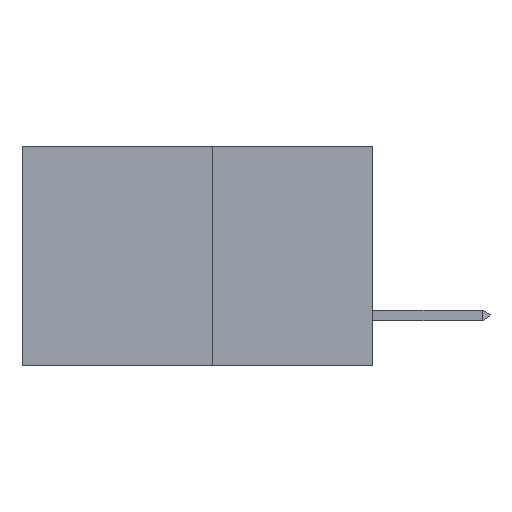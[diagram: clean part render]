
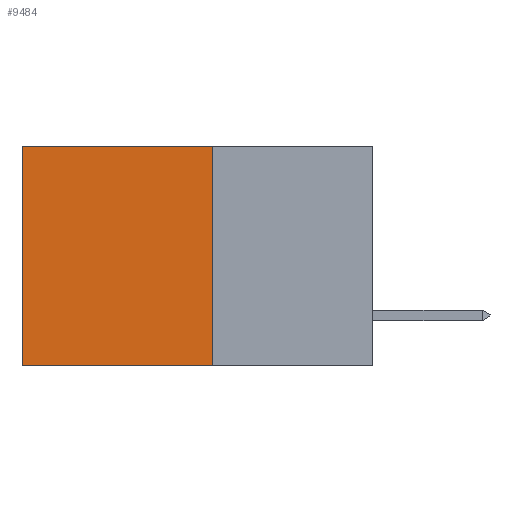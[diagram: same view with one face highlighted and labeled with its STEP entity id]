
A CAD part, left-side view. The second image highlights one B-rep face of the part: STEP entity #9484.
In plain terms, the highlighted planar face has unit normal (-1, 0, 0).
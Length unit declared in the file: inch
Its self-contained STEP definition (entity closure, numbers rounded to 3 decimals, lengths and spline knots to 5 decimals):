
#1274 = VERTEX_POINT ( 'NONE', #1843 ) ;
#1649 = DIRECTION ( 'NONE',  ( 0., 0., -1. ) ) ;
#1843 = CARTESIAN_POINT ( 'NONE',  ( 0.277, 0.59, 0. ) ) ;
#2267 = ORIENTED_EDGE ( 'NONE', *, *, #2368, .T. ) ;
#2368 = EDGE_CURVE ( 'NONE', #1274, #11305, #2535, .T. ) ;
#2535 = LINE ( 'NONE', #3333, #8054 ) ;
#2747 = CARTESIAN_POINT ( 'NONE',  ( 0.277, 0.27, -0.37 ) ) ;
#3224 = VECTOR ( 'NONE', #6146, 39.37008 ) ;
#3256 = DIRECTION ( 'NONE',  ( 0., 0., -1. ) ) ;
#3333 = CARTESIAN_POINT ( 'NONE',  ( 0.277, 0.59, -0.37 ) ) ;
#3532 = ORIENTED_EDGE ( 'NONE', *, *, #5782, .F. ) ;
#3908 = PLANE ( 'NONE',  #11185 ) ;
#4056 = CARTESIAN_POINT ( 'NONE',  ( 0.277, 0.59, -0.37 ) ) ;
#4429 = CARTESIAN_POINT ( 'NONE',  ( 0.277, 0.27, 0. ) ) ;
#4653 = LINE ( 'NONE', #7934, #12880 ) ;
#5021 = DIRECTION ( 'NONE',  ( 0., 0., -1. ) ) ;
#5252 = ORIENTED_EDGE ( 'NONE', *, *, #12631, .T. ) ;
#5782 = EDGE_CURVE ( 'NONE', #5898, #9797, #6721, .T. ) ;
#5898 = VERTEX_POINT ( 'NONE', #4429 ) ;
#6146 = DIRECTION ( 'NONE',  ( 0., 1., 0. ) ) ;
#6352 = EDGE_CURVE ( 'NONE', #9797, #11305, #4653, .T. ) ;
#6721 = LINE ( 'NONE', #8979, #7065 ) ;
#7065 = VECTOR ( 'NONE', #3256, 39.37008 ) ;
#7934 = CARTESIAN_POINT ( 'NONE',  ( 0.277, 0.27, -0.37 ) ) ;
#7975 = DIRECTION ( 'NONE',  ( 0., 1., 0. ) ) ;
#8054 = VECTOR ( 'NONE', #1649, 39.37008 ) ;
#8256 = EDGE_LOOP ( 'NONE', ( #2267, #11848, #3532, #5252 ) ) ;
#8979 = CARTESIAN_POINT ( 'NONE',  ( 0.277, 0.27, -0.37 ) ) ;
#9484 = ADVANCED_FACE ( 'NONE', ( #11998 ), #3908, .F. ) ;
#9797 = VERTEX_POINT ( 'NONE', #11928 ) ;
#11185 = AXIS2_PLACEMENT_3D ( 'NONE', #2747, #11469, #5021 ) ;
#11305 = VERTEX_POINT ( 'NONE', #4056 ) ;
#11469 = DIRECTION ( 'NONE',  ( 1., 0., 0. ) ) ;
#11848 = ORIENTED_EDGE ( 'NONE', *, *, #6352, .F. ) ;
#11928 = CARTESIAN_POINT ( 'NONE',  ( 0.277, 0.27, -0.37 ) ) ;
#11998 = FACE_OUTER_BOUND ( 'NONE', #8256, .T. ) ;
#12566 = CARTESIAN_POINT ( 'NONE',  ( 0.277, 0.27, 0. ) ) ;
#12631 = EDGE_CURVE ( 'NONE', #5898, #1274, #13652, .T. ) ;
#12880 = VECTOR ( 'NONE', #7975, 39.37008 ) ;
#13652 = LINE ( 'NONE', #12566, #3224 ) ;
